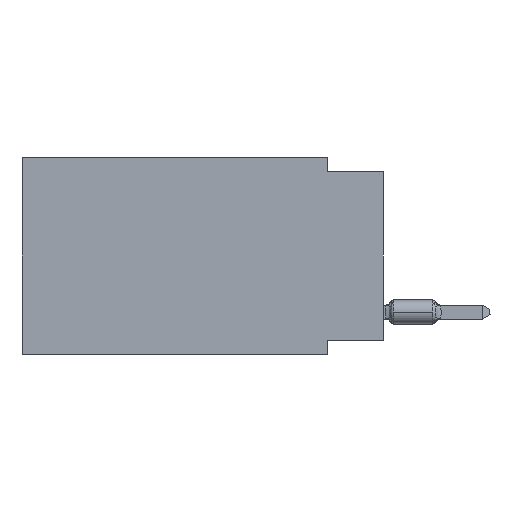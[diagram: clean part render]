
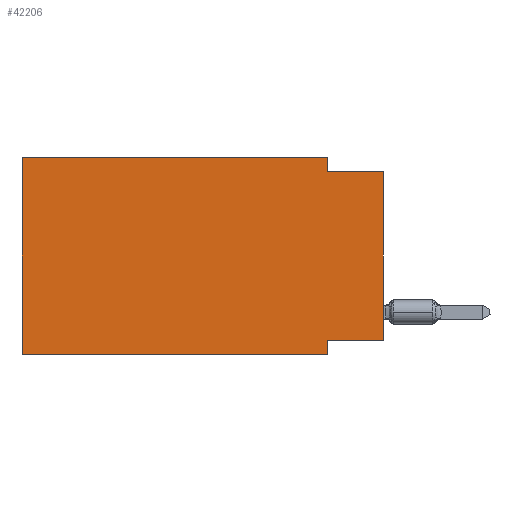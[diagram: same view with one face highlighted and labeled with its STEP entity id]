
A CAD part, left-side view. The second image highlights one B-rep face of the part: STEP entity #42206.
In plain terms, the highlighted planar face has unit normal (-1, 0, 0).
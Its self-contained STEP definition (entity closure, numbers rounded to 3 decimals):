
#915 = CARTESIAN_POINT ( 'NONE',  ( 0., 2.54, 0. ) ) ;
#1566 = CARTESIAN_POINT ( 'NONE',  ( 0., 0., -8.255 ) ) ;
#1640 = DIRECTION ( 'NONE',  ( 0., 0., -1. ) ) ;
#3291 = DIRECTION ( 'NONE',  ( 0., -1., 0. ) ) ;
#4057 = EDGE_CURVE ( 'NONE', #55328, #62214, #27807, .T. ) ;
#5141 = FACE_OUTER_BOUND ( 'NONE', #23798, .T. ) ;
#5551 = ORIENTED_EDGE ( 'NONE', *, *, #52637, .F. ) ;
#6803 = VERTEX_POINT ( 'NONE', #10831 ) ;
#8435 = CARTESIAN_POINT ( 'NONE',  ( 0., 0., -0.635 ) ) ;
#9532 = LINE ( 'NONE', #51838, #53792 ) ;
#10795 = LINE ( 'NONE', #69562, #44073 ) ;
#10831 = CARTESIAN_POINT ( 'NONE',  ( 0., 16.383, 0. ) ) ;
#10939 = ORIENTED_EDGE ( 'NONE', *, *, #43739, .F. ) ;
#14446 = CARTESIAN_POINT ( 'NONE',  ( 0., 2.54, -0.635 ) ) ;
#15082 = ORIENTED_EDGE ( 'NONE', *, *, #36861, .F. ) ;
#17767 = VECTOR ( 'NONE', #63240, 1000. ) ;
#19522 = CARTESIAN_POINT ( 'NONE',  ( 0., 16.383, 0. ) ) ;
#21957 = DIRECTION ( 'NONE',  ( 0., 0., -1. ) ) ;
#23798 = EDGE_LOOP ( 'NONE', ( #25148, #59792, #69444, #15082, #36232, #61542, #10939, #5551 ) ) ;
#24317 = VECTOR ( 'NONE', #1640, 1000. ) ;
#24893 = LINE ( 'NONE', #19522, #17767 ) ;
#25148 = ORIENTED_EDGE ( 'NONE', *, *, #27702, .T. ) ;
#25237 = CARTESIAN_POINT ( 'NONE',  ( 0., 16.383, -8.89 ) ) ;
#25579 = CARTESIAN_POINT ( 'NONE',  ( 0., 16.383, 0. ) ) ;
#27236 = LINE ( 'NONE', #33305, #50332 ) ;
#27702 = EDGE_CURVE ( 'NONE', #50463, #27838, #61506, .T. ) ;
#27807 = LINE ( 'NONE', #915, #24317 ) ;
#27838 = VERTEX_POINT ( 'NONE', #8435 ) ;
#28050 = LINE ( 'NONE', #44182, #34409 ) ;
#31238 = CARTESIAN_POINT ( 'NONE',  ( 0., 0., -0.635 ) ) ;
#31587 = VECTOR ( 'NONE', #3291, 1000. ) ;
#31752 = CARTESIAN_POINT ( 'NONE',  ( 0., 2.54, -8.255 ) ) ;
#32607 = DIRECTION ( 'NONE',  ( 0., -1., 0. ) ) ;
#33305 = CARTESIAN_POINT ( 'NONE',  ( 0., 16.383, -8.89 ) ) ;
#34409 = VECTOR ( 'NONE', #21957, 1000. ) ;
#36232 = ORIENTED_EDGE ( 'NONE', *, *, #46458, .F. ) ;
#36861 = EDGE_CURVE ( 'NONE', #6803, #55328, #24893, .T. ) ;
#36919 = CARTESIAN_POINT ( 'NONE',  ( 0., 2.54, 0. ) ) ;
#36981 = DIRECTION ( 'NONE',  ( 0., 0., 1. ) ) ;
#42206 = ADVANCED_FACE ( 'NONE', ( #5141 ), #48163, .F. ) ;
#43739 = EDGE_CURVE ( 'NONE', #47629, #50877, #28050, .T. ) ;
#44073 = VECTOR ( 'NONE', #36981, 1000. ) ;
#44182 = CARTESIAN_POINT ( 'NONE',  ( 0., 2.54, -8.89 ) ) ;
#46458 = EDGE_CURVE ( 'NONE', #65159, #6803, #10795, .T. ) ;
#47629 = VERTEX_POINT ( 'NONE', #31752 ) ;
#48163 = PLANE ( 'NONE',  #66473 ) ;
#50332 = VECTOR ( 'NONE', #32607, 1000. ) ;
#50463 = VERTEX_POINT ( 'NONE', #1566 ) ;
#50877 = VERTEX_POINT ( 'NONE', #67394 ) ;
#51838 = CARTESIAN_POINT ( 'NONE',  ( 0., 0., -8.255 ) ) ;
#52020 = EDGE_CURVE ( 'NONE', #65159, #50877, #27236, .T. ) ;
#52637 = EDGE_CURVE ( 'NONE', #50463, #47629, #9532, .T. ) ;
#53257 = DIRECTION ( 'NONE',  ( 0., 1., 0. ) ) ;
#53792 = VECTOR ( 'NONE', #53257, 1000. ) ;
#54441 = VECTOR ( 'NONE', #60792, 1000. ) ;
#55328 = VERTEX_POINT ( 'NONE', #36919 ) ;
#57077 = LINE ( 'NONE', #31238, #31587 ) ;
#59264 = DIRECTION ( 'NONE',  ( 0., 0., -1. ) ) ;
#59792 = ORIENTED_EDGE ( 'NONE', *, *, #68035, .F. ) ;
#60792 = DIRECTION ( 'NONE',  ( 0., 0., 1. ) ) ;
#61506 = LINE ( 'NONE', #67224, #54441 ) ;
#61542 = ORIENTED_EDGE ( 'NONE', *, *, #52020, .T. ) ;
#62214 = VERTEX_POINT ( 'NONE', #14446 ) ;
#63240 = DIRECTION ( 'NONE',  ( 0., -1., 0. ) ) ;
#64286 = DIRECTION ( 'NONE',  ( 1., 0., 0. ) ) ;
#65159 = VERTEX_POINT ( 'NONE', #25237 ) ;
#66473 = AXIS2_PLACEMENT_3D ( 'NONE', #25579, #64286, #59264 ) ;
#67224 = CARTESIAN_POINT ( 'NONE',  ( 0., 0., 0. ) ) ;
#67394 = CARTESIAN_POINT ( 'NONE',  ( 0., 2.54, -8.89 ) ) ;
#68035 = EDGE_CURVE ( 'NONE', #62214, #27838, #57077, .T. ) ;
#69444 = ORIENTED_EDGE ( 'NONE', *, *, #4057, .F. ) ;
#69562 = CARTESIAN_POINT ( 'NONE',  ( 0., 16.383, 0. ) ) ;
